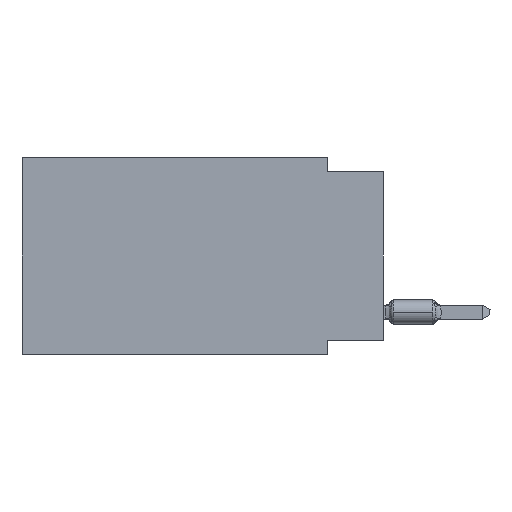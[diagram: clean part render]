
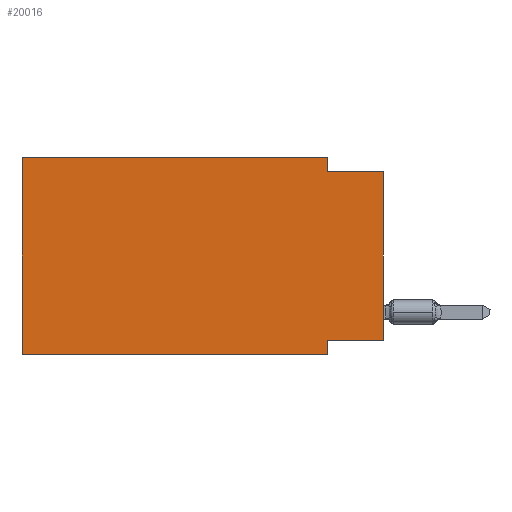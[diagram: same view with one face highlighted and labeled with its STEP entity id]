
A CAD part, left-side view. The second image highlights one B-rep face of the part: STEP entity #20016.
In plain terms, the highlighted planar face has unit normal (-1, 0, 0).
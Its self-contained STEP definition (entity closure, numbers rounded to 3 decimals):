
#589 = AXIS2_PLACEMENT_3D ( 'NONE', #21131, #20615, #12872 ) ;
#761 = CARTESIAN_POINT ( 'NONE',  ( 0., 2.54, 0. ) ) ;
#868 = LINE ( 'NONE', #4091, #5149 ) ;
#1405 = CARTESIAN_POINT ( 'NONE',  ( 0., 2.54, -8.89 ) ) ;
#1644 = VERTEX_POINT ( 'NONE', #20688 ) ;
#1713 = CARTESIAN_POINT ( 'NONE',  ( 0., 16.383, 0. ) ) ;
#1798 = CARTESIAN_POINT ( 'NONE',  ( 0., 2.54, -0.635 ) ) ;
#1963 = LINE ( 'NONE', #16750, #13443 ) ;
#2295 = VECTOR ( 'NONE', #19840, 1000. ) ;
#2653 = EDGE_CURVE ( 'NONE', #19431, #1644, #13221, .T. ) ;
#3040 = ORIENTED_EDGE ( 'NONE', *, *, #7104, .F. ) ;
#3144 = ORIENTED_EDGE ( 'NONE', *, *, #8901, .T. ) ;
#3522 = CARTESIAN_POINT ( 'NONE',  ( 0., 16.383, -8.89 ) ) ;
#4091 = CARTESIAN_POINT ( 'NONE',  ( 0., 2.54, 0. ) ) ;
#4301 = EDGE_CURVE ( 'NONE', #16003, #14793, #20575, .T. ) ;
#4529 = ORIENTED_EDGE ( 'NONE', *, *, #4658, .F. ) ;
#4658 = EDGE_CURVE ( 'NONE', #14793, #10744, #5132, .T. ) ;
#4768 = DIRECTION ( 'NONE',  ( 0., -1., 0. ) ) ;
#4783 = LINE ( 'NONE', #13245, #11726 ) ;
#4793 = ORIENTED_EDGE ( 'NONE', *, *, #2653, .F. ) ;
#5132 = LINE ( 'NONE', #1713, #8518 ) ;
#5149 = VECTOR ( 'NONE', #13735, 1000. ) ;
#5596 = DIRECTION ( 'NONE',  ( 0., 0., 1. ) ) ;
#7104 = EDGE_CURVE ( 'NONE', #19367, #14896, #4783, .T. ) ;
#7868 = LINE ( 'NONE', #1405, #9024 ) ;
#7964 = DIRECTION ( 'NONE',  ( 0., 0., -1. ) ) ;
#7973 = VERTEX_POINT ( 'NONE', #16413 ) ;
#8260 = DIRECTION ( 'NONE',  ( 0., -1., 0. ) ) ;
#8518 = VECTOR ( 'NONE', #8260, 1000. ) ;
#8901 = EDGE_CURVE ( 'NONE', #19431, #14896, #1963, .T. ) ;
#9024 = VECTOR ( 'NONE', #7964, 1000. ) ;
#10467 = CARTESIAN_POINT ( 'NONE',  ( 0., 0., -0.635 ) ) ;
#10743 = EDGE_CURVE ( 'NONE', #10744, #19367, #868, .T. ) ;
#10744 = VERTEX_POINT ( 'NONE', #761 ) ;
#10753 = ORIENTED_EDGE ( 'NONE', *, *, #10743, .F. ) ;
#11669 = CARTESIAN_POINT ( 'NONE',  ( 0., 16.383, 0. ) ) ;
#11726 = VECTOR ( 'NONE', #17633, 1000. ) ;
#12872 = DIRECTION ( 'NONE',  ( 0., 0., -1. ) ) ;
#13221 = LINE ( 'NONE', #14932, #2295 ) ;
#13245 = CARTESIAN_POINT ( 'NONE',  ( 0., 0., -0.635 ) ) ;
#13443 = VECTOR ( 'NONE', #5596, 1000. ) ;
#13713 = CARTESIAN_POINT ( 'NONE',  ( 0., 16.383, 0. ) ) ;
#13735 = DIRECTION ( 'NONE',  ( 0., 0., -1. ) ) ;
#13976 = VECTOR ( 'NONE', #17037, 1000. ) ;
#14086 = PLANE ( 'NONE',  #589 ) ;
#14299 = EDGE_CURVE ( 'NONE', #1644, #7973, #7868, .T. ) ;
#14527 = CARTESIAN_POINT ( 'NONE',  ( 0., 16.383, -8.89 ) ) ;
#14738 = LINE ( 'NONE', #14527, #18632 ) ;
#14793 = VERTEX_POINT ( 'NONE', #11669 ) ;
#14896 = VERTEX_POINT ( 'NONE', #10467 ) ;
#14932 = CARTESIAN_POINT ( 'NONE',  ( 0., 0., -8.255 ) ) ;
#15108 = ORIENTED_EDGE ( 'NONE', *, *, #15574, .T. ) ;
#15574 = EDGE_CURVE ( 'NONE', #16003, #7973, #14738, .T. ) ;
#16003 = VERTEX_POINT ( 'NONE', #3522 ) ;
#16087 = EDGE_LOOP ( 'NONE', ( #3144, #3040, #10753, #4529, #17737, #15108, #20201, #4793 ) ) ;
#16413 = CARTESIAN_POINT ( 'NONE',  ( 0., 2.54, -8.89 ) ) ;
#16750 = CARTESIAN_POINT ( 'NONE',  ( 0., 0., 0. ) ) ;
#17037 = DIRECTION ( 'NONE',  ( 0., 0., 1. ) ) ;
#17293 = FACE_OUTER_BOUND ( 'NONE', #16087, .T. ) ;
#17633 = DIRECTION ( 'NONE',  ( 0., -1., 0. ) ) ;
#17737 = ORIENTED_EDGE ( 'NONE', *, *, #4301, .F. ) ;
#18181 = CARTESIAN_POINT ( 'NONE',  ( 0., 0., -8.255 ) ) ;
#18632 = VECTOR ( 'NONE', #4768, 1000. ) ;
#19367 = VERTEX_POINT ( 'NONE', #1798 ) ;
#19431 = VERTEX_POINT ( 'NONE', #18181 ) ;
#19840 = DIRECTION ( 'NONE',  ( 0., 1., 0. ) ) ;
#20016 = ADVANCED_FACE ( 'NONE', ( #17293 ), #14086, .F. ) ;
#20201 = ORIENTED_EDGE ( 'NONE', *, *, #14299, .F. ) ;
#20575 = LINE ( 'NONE', #13713, #13976 ) ;
#20615 = DIRECTION ( 'NONE',  ( 1., 0., 0. ) ) ;
#20688 = CARTESIAN_POINT ( 'NONE',  ( 0., 2.54, -8.255 ) ) ;
#21131 = CARTESIAN_POINT ( 'NONE',  ( 0., 16.383, 0. ) ) ;
